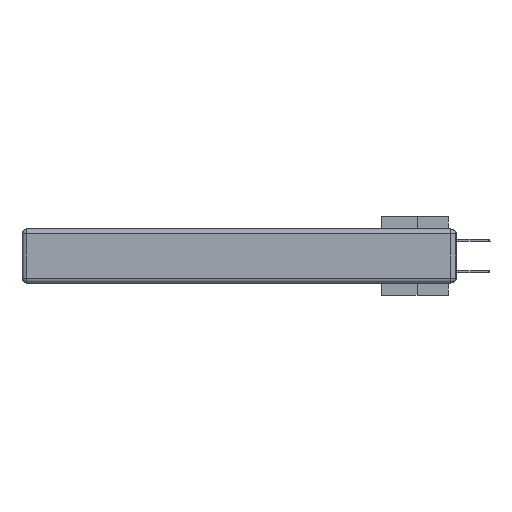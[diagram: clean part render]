
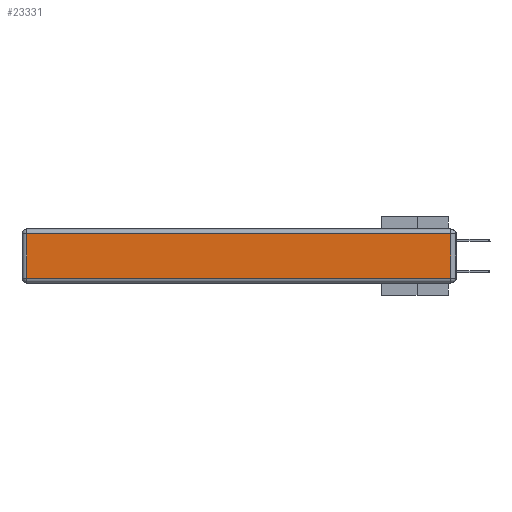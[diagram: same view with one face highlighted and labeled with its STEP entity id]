
A CAD part, left-side view. The second image highlights one B-rep face of the part: STEP entity #23331.
In plain terms, the highlighted planar face has unit normal (-1, 0, 0).
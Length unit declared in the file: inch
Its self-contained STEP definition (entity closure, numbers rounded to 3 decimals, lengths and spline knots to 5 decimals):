
#1488 = EDGE_CURVE ( 'NONE', #6287, #6550, #36101, .T. ) ;
#2281 = VECTOR ( 'NONE', #34835, 39.37008 ) ;
#2321 = CARTESIAN_POINT ( 'NONE',  ( 0., 0.03, -0.313 ) ) ;
#3071 = VECTOR ( 'NONE', #28397, 39.37008 ) ;
#4340 = EDGE_LOOP ( 'NONE', ( #13055, #16432, #10098, #23924 ) ) ;
#5754 = FACE_OUTER_BOUND ( 'NONE', #4340, .T. ) ;
#6287 = VERTEX_POINT ( 'NONE', #28442 ) ;
#6437 = EDGE_CURVE ( 'NONE', #19633, #6287, #9678, .T. ) ;
#6550 = VERTEX_POINT ( 'NONE', #2321 ) ;
#7454 = CARTESIAN_POINT ( 'NONE',  ( 0., 2.75, -0.03 ) ) ;
#8702 = DIRECTION ( 'NONE',  ( -1., 0., 0. ) ) ;
#9678 = LINE ( 'NONE', #23994, #25334 ) ;
#10098 = ORIENTED_EDGE ( 'NONE', *, *, #21139, .T. ) ;
#10610 = CARTESIAN_POINT ( 'NONE',  ( 0., 0.03, -0.343 ) ) ;
#12600 = DIRECTION ( 'NONE',  ( 0., 0., -1. ) ) ;
#12940 = VERTEX_POINT ( 'NONE', #28578 ) ;
#13055 = ORIENTED_EDGE ( 'NONE', *, *, #1488, .T. ) ;
#15088 = VECTOR ( 'NONE', #21980, 39.37008 ) ;
#16432 = ORIENTED_EDGE ( 'NONE', *, *, #17610, .T. ) ;
#17610 = EDGE_CURVE ( 'NONE', #6550, #12940, #32833, .T. ) ;
#19633 = VERTEX_POINT ( 'NONE', #20637 ) ;
#20253 = PLANE ( 'NONE',  #26801 ) ;
#20637 = CARTESIAN_POINT ( 'NONE',  ( 0., 2.72, -0.03 ) ) ;
#21139 = EDGE_CURVE ( 'NONE', #12940, #19633, #21233, .T. ) ;
#21233 = LINE ( 'NONE', #7454, #2281 ) ;
#21980 = DIRECTION ( 'NONE',  ( 0., 0., 1. ) ) ;
#22681 = CARTESIAN_POINT ( 'NONE',  ( 0., 0., -0.313 ) ) ;
#23331 = ADVANCED_FACE ( 'NONE', ( #5754 ), #20253, .T. ) ;
#23924 = ORIENTED_EDGE ( 'NONE', *, *, #6437, .T. ) ;
#23994 = CARTESIAN_POINT ( 'NONE',  ( 0., 2.72, -0.343 ) ) ;
#25334 = VECTOR ( 'NONE', #12600, 39.37008 ) ;
#26801 = AXIS2_PLACEMENT_3D ( 'NONE', #33690, #8702, #31298 ) ;
#28397 = DIRECTION ( 'NONE',  ( 0., -1., 0. ) ) ;
#28442 = CARTESIAN_POINT ( 'NONE',  ( 0., 2.72, -0.313 ) ) ;
#28578 = CARTESIAN_POINT ( 'NONE',  ( 0., 0.03, -0.03 ) ) ;
#31298 = DIRECTION ( 'NONE',  ( 0., 0., 1. ) ) ;
#32833 = LINE ( 'NONE', #10610, #15088 ) ;
#33690 = CARTESIAN_POINT ( 'NONE',  ( 0., 0., -0.343 ) ) ;
#34835 = DIRECTION ( 'NONE',  ( 0., 1., 0. ) ) ;
#36101 = LINE ( 'NONE', #22681, #3071 ) ;
